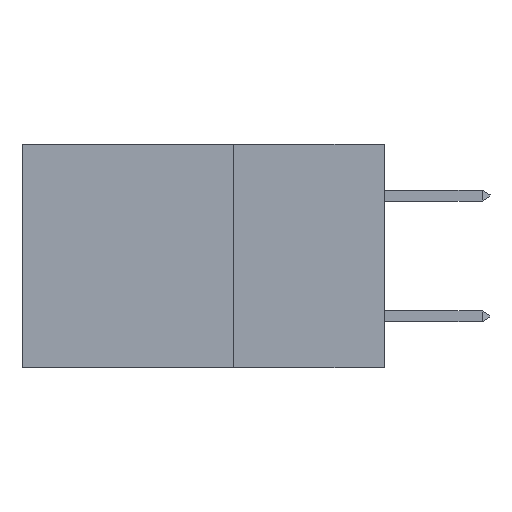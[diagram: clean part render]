
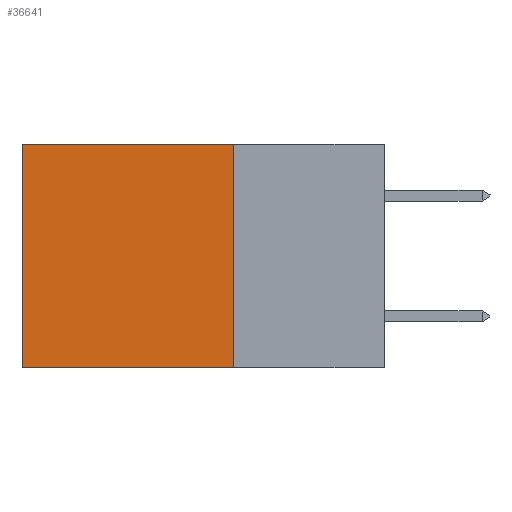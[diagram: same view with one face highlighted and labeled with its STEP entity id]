
A CAD part, left-side view. The second image highlights one B-rep face of the part: STEP entity #36641.
In plain terms, the highlighted planar face has unit normal (-1, 0, 0).
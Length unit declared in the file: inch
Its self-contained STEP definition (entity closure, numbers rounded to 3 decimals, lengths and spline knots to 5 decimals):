
#14 = PLANE ( 'NONE',  #39813 ) ;
#1827 = ORIENTED_EDGE ( 'NONE', *, *, #11317, .F. ) ;
#2754 = DIRECTION ( 'NONE',  ( 0., 0., -1. ) ) ;
#3403 = VECTOR ( 'NONE', #33663, 39.37008 ) ;
#3653 = CARTESIAN_POINT ( 'NONE',  ( 0.2875, 0.6, 0. ) ) ;
#6053 = CARTESIAN_POINT ( 'NONE',  ( 0.2875, 0.25, -0.37 ) ) ;
#6276 = CARTESIAN_POINT ( 'NONE',  ( 0.2875, 0.25, 0. ) ) ;
#6990 = VECTOR ( 'NONE', #14252, 39.37008 ) ;
#9024 = DIRECTION ( 'NONE',  ( 1., 0., 0. ) ) ;
#9080 = EDGE_CURVE ( 'NONE', #11574, #30611, #25575, .T. ) ;
#9431 = LINE ( 'NONE', #6053, #40339 ) ;
#10677 = CARTESIAN_POINT ( 'NONE',  ( 0.2875, 0.25, 0. ) ) ;
#11317 = EDGE_CURVE ( 'NONE', #17012, #15123, #14422, .T. ) ;
#11340 = CARTESIAN_POINT ( 'NONE',  ( 0.2875, 0.25, 0. ) ) ;
#11574 = VERTEX_POINT ( 'NONE', #3653 ) ;
#14252 = DIRECTION ( 'NONE',  ( 0., 1., 0. ) ) ;
#14422 = LINE ( 'NONE', #34847, #3403 ) ;
#15123 = VERTEX_POINT ( 'NONE', #28768 ) ;
#17012 = VERTEX_POINT ( 'NONE', #10677 ) ;
#18834 = DIRECTION ( 'NONE',  ( 0., 1., 0. ) ) ;
#18883 = CARTESIAN_POINT ( 'NONE',  ( 0.2875, 0.6, 0. ) ) ;
#19407 = VECTOR ( 'NONE', #2754, 39.37008 ) ;
#20950 = LINE ( 'NONE', #11340, #6990 ) ;
#21035 = ORIENTED_EDGE ( 'NONE', *, *, #9080, .T. ) ;
#25575 = LINE ( 'NONE', #18883, #19407 ) ;
#28060 = FACE_OUTER_BOUND ( 'NONE', #31259, .T. ) ;
#28353 = ORIENTED_EDGE ( 'NONE', *, *, #35207, .T. ) ;
#28697 = DIRECTION ( 'NONE',  ( 0., 0., -1. ) ) ;
#28768 = CARTESIAN_POINT ( 'NONE',  ( 0.2875, 0.25, -0.37 ) ) ;
#30611 = VERTEX_POINT ( 'NONE', #37490 ) ;
#31259 = EDGE_LOOP ( 'NONE', ( #21035, #39350, #1827, #28353 ) ) ;
#33663 = DIRECTION ( 'NONE',  ( 0., 0., -1. ) ) ;
#34000 = EDGE_CURVE ( 'NONE', #15123, #30611, #9431, .T. ) ;
#34847 = CARTESIAN_POINT ( 'NONE',  ( 0.2875, 0.25, 0. ) ) ;
#35207 = EDGE_CURVE ( 'NONE', #17012, #11574, #20950, .T. ) ;
#36641 = ADVANCED_FACE ( 'NONE', ( #28060 ), #14, .F. ) ;
#37490 = CARTESIAN_POINT ( 'NONE',  ( 0.2875, 0.6, -0.37 ) ) ;
#39350 = ORIENTED_EDGE ( 'NONE', *, *, #34000, .F. ) ;
#39813 = AXIS2_PLACEMENT_3D ( 'NONE', #6276, #9024, #28697 ) ;
#40339 = VECTOR ( 'NONE', #18834, 39.37008 ) ;
